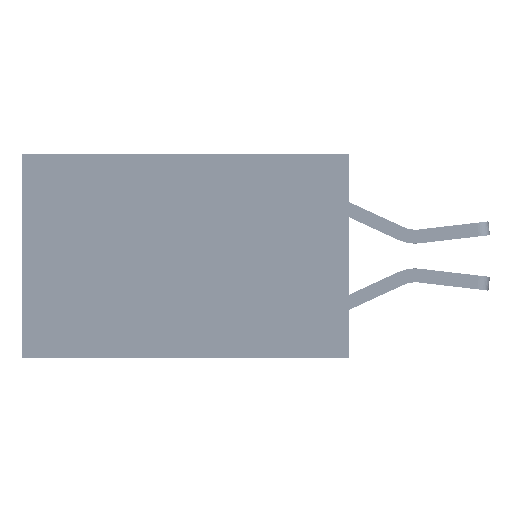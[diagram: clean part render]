
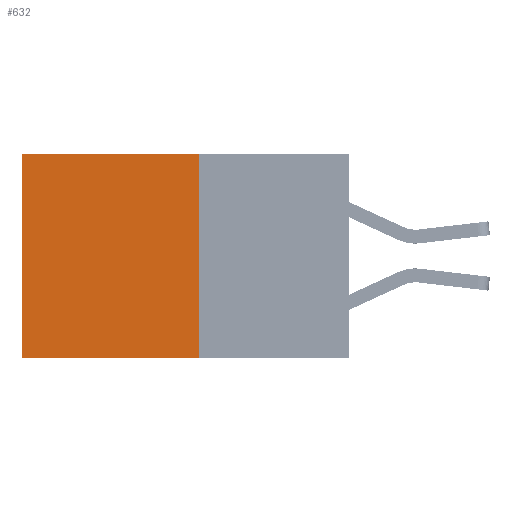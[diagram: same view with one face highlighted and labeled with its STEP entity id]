
A CAD part, left-side view. The second image highlights one B-rep face of the part: STEP entity #632.
In plain terms, the highlighted planar face has unit normal (-1, 0, 0).
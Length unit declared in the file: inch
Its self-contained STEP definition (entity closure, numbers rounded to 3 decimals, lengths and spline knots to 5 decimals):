
#632 = ADVANCED_FACE ( 'NONE', ( #11291 ), #23407, .F. ) ;
#1104 = CARTESIAN_POINT ( 'NONE',  ( 0.277, 0.27, -0.37 ) ) ;
#1443 = ORIENTED_EDGE ( 'NONE', *, *, #8614, .T. ) ;
#1936 = DIRECTION ( 'NONE',  ( 0., 1., 0. ) ) ;
#4868 = VECTOR ( 'NONE', #19256, 39.37008 ) ;
#6473 = CARTESIAN_POINT ( 'NONE',  ( 0.277, 0.27, 0. ) ) ;
#7953 = CARTESIAN_POINT ( 'NONE',  ( 0.277, 0.27, -0.37 ) ) ;
#8404 = VECTOR ( 'NONE', #13319, 39.37008 ) ;
#8406 = LINE ( 'NONE', #7953, #28611 ) ;
#8614 = EDGE_CURVE ( 'NONE', #27321, #19818, #11350, .T. ) ;
#8897 = ORIENTED_EDGE ( 'NONE', *, *, #12990, .F. ) ;
#10292 = CARTESIAN_POINT ( 'NONE',  ( 0.277, 0.27, 0. ) ) ;
#10498 = CARTESIAN_POINT ( 'NONE',  ( 0.277, 0.27, -0.37 ) ) ;
#11291 = FACE_OUTER_BOUND ( 'NONE', #21235, .T. ) ;
#11350 = LINE ( 'NONE', #10292, #18688 ) ;
#12990 = EDGE_CURVE ( 'NONE', #27321, #18585, #30304, .T. ) ;
#13319 = DIRECTION ( 'NONE',  ( 0., 0., -1. ) ) ;
#16980 = CARTESIAN_POINT ( 'NONE',  ( 0.277, 0.59, -0.37 ) ) ;
#18585 = VERTEX_POINT ( 'NONE', #1104 ) ;
#18688 = VECTOR ( 'NONE', #1936, 39.37008 ) ;
#19256 = DIRECTION ( 'NONE',  ( 0., 0., -1. ) ) ;
#19411 = AXIS2_PLACEMENT_3D ( 'NONE', #22475, #23107, #23332 ) ;
#19818 = VERTEX_POINT ( 'NONE', #24333 ) ;
#21235 = EDGE_LOOP ( 'NONE', ( #21573, #33281, #8897, #1443 ) ) ;
#21573 = ORIENTED_EDGE ( 'NONE', *, *, #33914, .T. ) ;
#21837 = EDGE_CURVE ( 'NONE', #18585, #23746, #8406, .T. ) ;
#22475 = CARTESIAN_POINT ( 'NONE',  ( 0.277, 0.27, -0.37 ) ) ;
#23107 = DIRECTION ( 'NONE',  ( 1., 0., 0. ) ) ;
#23332 = DIRECTION ( 'NONE',  ( 0., 0., -1. ) ) ;
#23407 = PLANE ( 'NONE',  #19411 ) ;
#23746 = VERTEX_POINT ( 'NONE', #16980 ) ;
#24333 = CARTESIAN_POINT ( 'NONE',  ( 0.277, 0.59, 0. ) ) ;
#27321 = VERTEX_POINT ( 'NONE', #6473 ) ;
#28611 = VECTOR ( 'NONE', #35405, 39.37008 ) ;
#30304 = LINE ( 'NONE', #10498, #8404 ) ;
#32858 = CARTESIAN_POINT ( 'NONE',  ( 0.277, 0.59, -0.37 ) ) ;
#33235 = LINE ( 'NONE', #32858, #4868 ) ;
#33281 = ORIENTED_EDGE ( 'NONE', *, *, #21837, .F. ) ;
#33914 = EDGE_CURVE ( 'NONE', #19818, #23746, #33235, .T. ) ;
#35405 = DIRECTION ( 'NONE',  ( 0., 1., 0. ) ) ;
